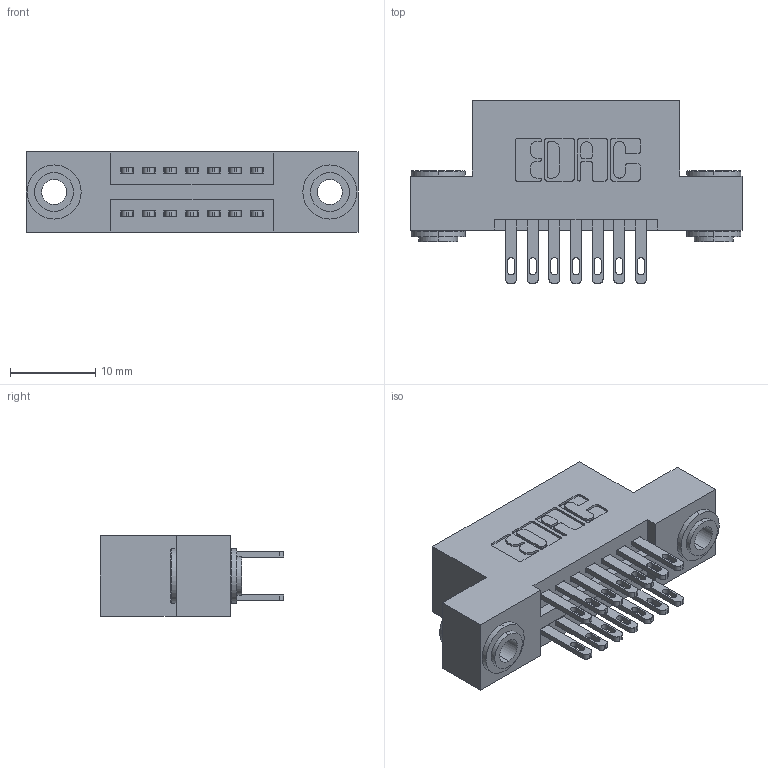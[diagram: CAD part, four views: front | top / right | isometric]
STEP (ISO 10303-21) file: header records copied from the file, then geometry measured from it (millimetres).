
FILE_DESCRIPTION (( 'STEP AP203' ), '1' );
FILE_NAME ('895-014-500-203.STEP', '2020-09-25T02:45:42', ( '' ), ( '' ), 'SwSTEP 2.0', 'SolidWorks 2020', '' );
FILE_SCHEMA (( 'CONFIG_CONTROL_DESIGN' ));
Length unit declared in the file: inch
Products named in the file (4): 845 Part_Flush Mounting Lugs - 0.156 Dia-TH; 895-014-500-203; 345-292-001_345-293-100; 345-250-002_345-250-002-102
Assembly tree (17 placements, depth 2):
  895-014-500-203
    845 Part_Flush Mounting Lugs - 0.156 Dia-TH
    345-292-001_345-293-100  x14
    345-250-002_345-250-002-102  x2
Bounding box: 38.99 x 21.51 x 9.4 mm (x, y, z)
Volume: 3524.7 mm3; surface area: 4879.9 mm2
Topology: 17 solids, 17 shells, 808 faces, 2391 edges, 1590 vertices
Faces by surface type: plane 468, cylinder 332, cone 8
Entity records: 10784 total; most frequent: CARTESIAN_POINT 1815, ORIENTED_EDGE 1742, DIRECTION 1677, EDGE_CURVE 871, LINE 683, VECTOR 683, VERTEX_POINT 578, AXIS2_PLACEMENT_3D 497
